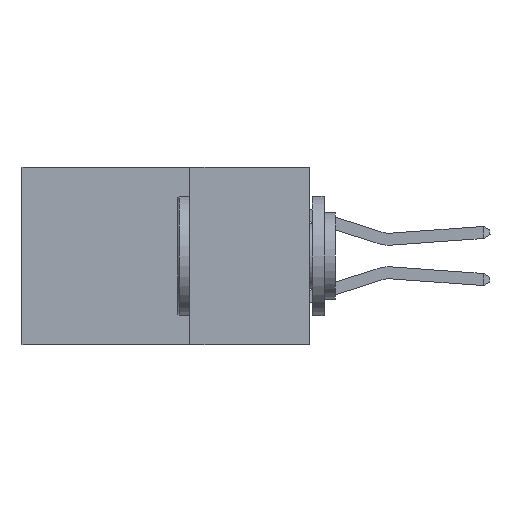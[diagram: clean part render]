
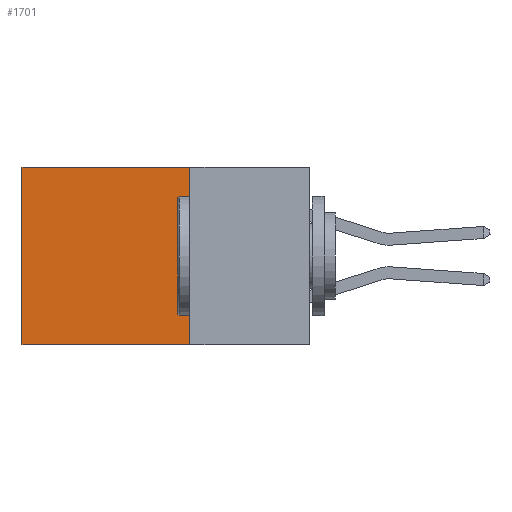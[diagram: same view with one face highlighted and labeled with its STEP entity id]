
A CAD part, left-side view. The second image highlights one B-rep face of the part: STEP entity #1701.
In plain terms, the highlighted planar face has unit normal (-1, 0, 0).
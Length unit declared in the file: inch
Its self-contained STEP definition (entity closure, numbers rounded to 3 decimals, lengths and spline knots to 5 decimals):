
#401 = CARTESIAN_POINT ( 'NONE',  ( 0.298, 0.6, 0. ) ) ;
#1701 = ADVANCED_FACE ( 'NONE', ( #14204 ), #4892, .F. ) ;
#1806 = DIRECTION ( 'NONE',  ( 0., 1., 0. ) ) ;
#2531 = LINE ( 'NONE', #11841, #18558 ) ;
#2724 = DIRECTION ( 'NONE',  ( 0., 0., -1. ) ) ;
#3046 = CARTESIAN_POINT ( 'NONE',  ( 0.298, 0.25, 0. ) ) ;
#4892 = PLANE ( 'NONE',  #17104 ) ;
#5174 = DIRECTION ( 'NONE',  ( 0., 0., -1. ) ) ;
#5768 = DIRECTION ( 'NONE',  ( 0., 0., -1. ) ) ;
#6196 = CARTESIAN_POINT ( 'NONE',  ( 0.298, 0.25, -0.37 ) ) ;
#6374 = CARTESIAN_POINT ( 'NONE',  ( 0.298, 0.25, -0.37 ) ) ;
#6832 = DIRECTION ( 'NONE',  ( 0., 1., 0. ) ) ;
#9356 = LINE ( 'NONE', #25451, #16115 ) ;
#9654 = EDGE_CURVE ( 'NONE', #17671, #12812, #10179, .T. ) ;
#10179 = LINE ( 'NONE', #6196, #23674 ) ;
#11558 = EDGE_CURVE ( 'NONE', #20727, #17671, #22475, .T. ) ;
#11841 = CARTESIAN_POINT ( 'NONE',  ( 0.298, 0.25, 0. ) ) ;
#12812 = VERTEX_POINT ( 'NONE', #26349 ) ;
#13218 = ORIENTED_EDGE ( 'NONE', *, *, #25380, .T. ) ;
#14204 = FACE_OUTER_BOUND ( 'NONE', #28931, .T. ) ;
#14362 = CARTESIAN_POINT ( 'NONE',  ( 0.298, 0.25, 0. ) ) ;
#15777 = ORIENTED_EDGE ( 'NONE', *, *, #26394, .T. ) ;
#16115 = VECTOR ( 'NONE', #5174, 39.37008 ) ;
#17104 = AXIS2_PLACEMENT_3D ( 'NONE', #14362, #25673, #2724 ) ;
#17671 = VERTEX_POINT ( 'NONE', #6374 ) ;
#18558 = VECTOR ( 'NONE', #6832, 39.37008 ) ;
#20727 = VERTEX_POINT ( 'NONE', #3046 ) ;
#21786 = VECTOR ( 'NONE', #5768, 39.37008 ) ;
#22112 = ORIENTED_EDGE ( 'NONE', *, *, #11558, .F. ) ;
#22475 = LINE ( 'NONE', #24234, #21786 ) ;
#23674 = VECTOR ( 'NONE', #1806, 39.37008 ) ;
#24234 = CARTESIAN_POINT ( 'NONE',  ( 0.298, 0.25, 0. ) ) ;
#25359 = VERTEX_POINT ( 'NONE', #401 ) ;
#25380 = EDGE_CURVE ( 'NONE', #25359, #12812, #9356, .T. ) ;
#25451 = CARTESIAN_POINT ( 'NONE',  ( 0.298, 0.6, 0. ) ) ;
#25673 = DIRECTION ( 'NONE',  ( 1., 0., 0. ) ) ;
#26349 = CARTESIAN_POINT ( 'NONE',  ( 0.298, 0.6, -0.37 ) ) ;
#26394 = EDGE_CURVE ( 'NONE', #20727, #25359, #2531, .T. ) ;
#27851 = ORIENTED_EDGE ( 'NONE', *, *, #9654, .F. ) ;
#28931 = EDGE_LOOP ( 'NONE', ( #13218, #27851, #22112, #15777 ) ) ;
